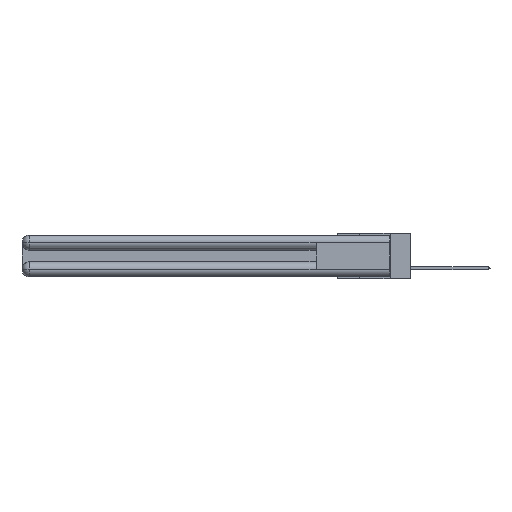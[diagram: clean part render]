
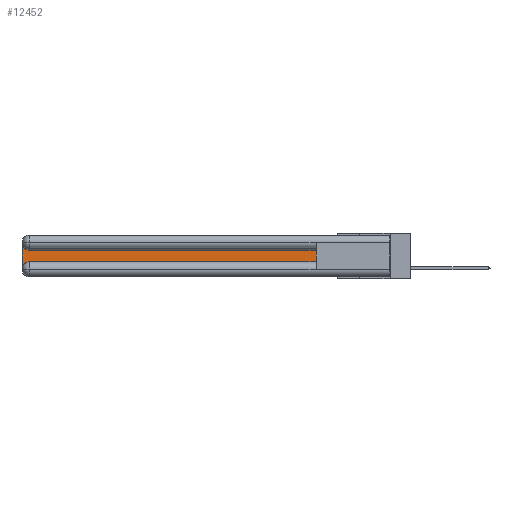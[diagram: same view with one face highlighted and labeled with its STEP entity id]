
A CAD part, left-side view. The second image highlights one B-rep face of the part: STEP entity #12452.
In plain terms, the highlighted planar face has unit normal (-1, 0, 0).
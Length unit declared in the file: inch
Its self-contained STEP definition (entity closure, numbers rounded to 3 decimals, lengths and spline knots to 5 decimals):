
#96 = DIRECTION ( 'NONE',  ( 1., 0., 0. ) ) ;
#373 = CIRCLE ( 'NONE', #6667, 0.06 ) ;
#401 = DIRECTION ( 'NONE',  ( 1., 0., 0. ) ) ;
#480 = VERTEX_POINT ( 'NONE', #9247 ) ;
#636 = FACE_OUTER_BOUND ( 'NONE', #11945, .T. ) ;
#1071 = CARTESIAN_POINT ( 'NONE',  ( 0.075, 0.6, -0.2175 ) ) ;
#1509 = DIRECTION ( 'NONE',  ( 0., 0., 1. ) ) ;
#1808 = EDGE_CURVE ( 'NONE', #20000, #26298, #14010, .T. ) ;
#2653 = ORIENTED_EDGE ( 'NONE', *, *, #1808, .T. ) ;
#5437 = DIRECTION ( 'NONE',  ( 0., 0., -1. ) ) ;
#5497 = CARTESIAN_POINT ( 'NONE',  ( 0.075, 0.6, -0.2175 ) ) ;
#6100 = EDGE_CURVE ( 'NONE', #23998, #480, #30194, .T. ) ;
#6667 = AXIS2_PLACEMENT_3D ( 'NONE', #27141, #12555, #29623 ) ;
#7668 = EDGE_CURVE ( 'NONE', #23903, #23217, #373, .T. ) ;
#8049 = CARTESIAN_POINT ( 'NONE',  ( 0.075, 3., -0.1225 ) ) ;
#8241 = ORIENTED_EDGE ( 'NONE', *, *, #25695, .T. ) ;
#9171 = AXIS2_PLACEMENT_3D ( 'NONE', #26669, #96, #21965 ) ;
#9247 = CARTESIAN_POINT ( 'NONE',  ( 0.075, 0.6, -0.1225 ) ) ;
#10271 = PLANE ( 'NONE',  #18249 ) ;
#10306 = VECTOR ( 'NONE', #21105, 39.37008 ) ;
#10562 = ORIENTED_EDGE ( 'NONE', *, *, #7668, .T. ) ;
#11945 = EDGE_LOOP ( 'NONE', ( #16813, #2653, #8241, #10562, #19506, #20479 ) ) ;
#12452 = ADVANCED_FACE ( 'NONE', ( #636 ), #10271, .F. ) ;
#12555 = DIRECTION ( 'NONE',  ( 1., 0., 0. ) ) ;
#14010 = CIRCLE ( 'NONE', #9171, 0.06 ) ;
#14528 = DIRECTION ( 'NONE',  ( 0., 0., -1. ) ) ;
#15134 = EDGE_CURVE ( 'NONE', #480, #20000, #28241, .T. ) ;
#15289 = CARTESIAN_POINT ( 'NONE',  ( 0.075, 2.94, -0.1225 ) ) ;
#15872 = LINE ( 'NONE', #5497, #20467 ) ;
#16087 = CARTESIAN_POINT ( 'NONE',  ( 0.075, 0.6, -0.1225 ) ) ;
#16813 = ORIENTED_EDGE ( 'NONE', *, *, #15134, .T. ) ;
#17425 = CARTESIAN_POINT ( 'NONE',  ( 0.075, 3., -0.0625 ) ) ;
#18249 = AXIS2_PLACEMENT_3D ( 'NONE', #8049, #401, #5437 ) ;
#18979 = LINE ( 'NONE', #28966, #28544 ) ;
#19239 = CARTESIAN_POINT ( 'NONE',  ( 0.075, 2.94, -0.2175 ) ) ;
#19417 = CARTESIAN_POINT ( 'NONE',  ( 0.075, 3., -0.2775 ) ) ;
#19506 = ORIENTED_EDGE ( 'NONE', *, *, #22362, .T. ) ;
#19991 = DIRECTION ( 'NONE',  ( 0., -1., 0. ) ) ;
#20000 = VERTEX_POINT ( 'NONE', #15289 ) ;
#20467 = VECTOR ( 'NONE', #19991, 39.37008 ) ;
#20479 = ORIENTED_EDGE ( 'NONE', *, *, #6100, .T. ) ;
#21105 = DIRECTION ( 'NONE',  ( 0., 1., 0. ) ) ;
#21965 = DIRECTION ( 'NONE',  ( 0., 0., -1. ) ) ;
#22362 = EDGE_CURVE ( 'NONE', #23217, #23998, #15872, .T. ) ;
#22797 = CARTESIAN_POINT ( 'NONE',  ( 0.075, 0.6, -0.2175 ) ) ;
#23217 = VERTEX_POINT ( 'NONE', #19239 ) ;
#23903 = VERTEX_POINT ( 'NONE', #19417 ) ;
#23998 = VERTEX_POINT ( 'NONE', #22797 ) ;
#25695 = EDGE_CURVE ( 'NONE', #26298, #23903, #18979, .T. ) ;
#26298 = VERTEX_POINT ( 'NONE', #17425 ) ;
#26332 = VECTOR ( 'NONE', #1509, 39.37008 ) ;
#26669 = CARTESIAN_POINT ( 'NONE',  ( 0.075, 2.94, -0.0625 ) ) ;
#27141 = CARTESIAN_POINT ( 'NONE',  ( 0.075, 2.94, -0.2775 ) ) ;
#28241 = LINE ( 'NONE', #16087, #10306 ) ;
#28544 = VECTOR ( 'NONE', #14528, 39.37008 ) ;
#28966 = CARTESIAN_POINT ( 'NONE',  ( 0.075, 3., -0.2175 ) ) ;
#29623 = DIRECTION ( 'NONE',  ( 0., 0., -1. ) ) ;
#30194 = LINE ( 'NONE', #1071, #26332 ) ;
